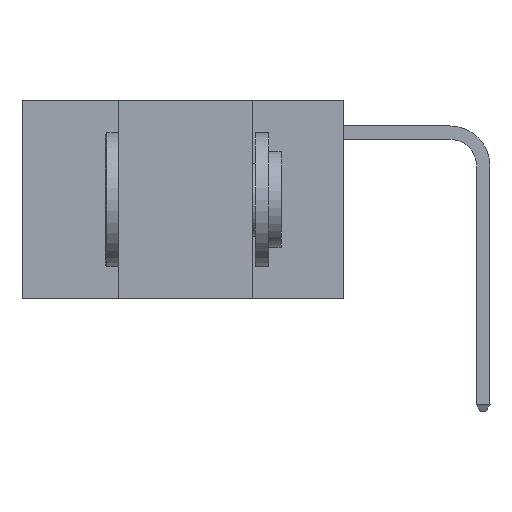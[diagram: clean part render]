
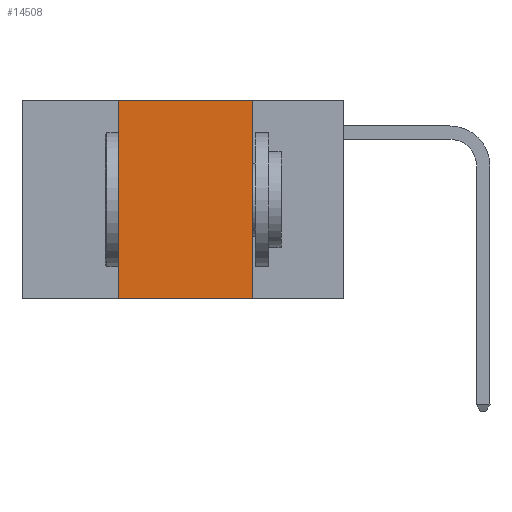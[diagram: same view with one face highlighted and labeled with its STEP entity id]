
A CAD part, left-side view. The second image highlights one B-rep face of the part: STEP entity #14508.
In plain terms, the highlighted planar face has unit normal (-1, 0, 0).
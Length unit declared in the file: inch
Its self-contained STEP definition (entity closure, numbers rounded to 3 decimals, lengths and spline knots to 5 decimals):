
#863 = DIRECTION ( 'NONE',  ( 0., -1., 0. ) ) ;
#2679 = LINE ( 'NONE', #19055, #10497 ) ;
#3425 = DIRECTION ( 'NONE',  ( 0., -1., 0. ) ) ;
#3497 = VECTOR ( 'NONE', #9899, 39.37008 ) ;
#4027 = CARTESIAN_POINT ( 'NONE',  ( 0., 0.6, -0.37 ) ) ;
#4130 = EDGE_LOOP ( 'NONE', ( #8446, #8509, #8854, #9112 ) ) ;
#4218 = VECTOR ( 'NONE', #3425, 39.37008 ) ;
#4928 = CARTESIAN_POINT ( 'NONE',  ( 0., 0.6, 0. ) ) ;
#6399 = DIRECTION ( 'NONE',  ( 0., 0., -1. ) ) ;
#6536 = CARTESIAN_POINT ( 'NONE',  ( 0., 0.17, 0. ) ) ;
#6576 = DIRECTION ( 'NONE',  ( 0., 0., -1. ) ) ;
#6963 = LINE ( 'NONE', #6536, #11026 ) ;
#8057 = PLANE ( 'NONE',  #15770 ) ;
#8110 = EDGE_CURVE ( 'NONE', #13884, #10195, #6963, .T. ) ;
#8275 = EDGE_CURVE ( 'NONE', #11967, #10195, #8441, .T. ) ;
#8441 = LINE ( 'NONE', #4027, #4218 ) ;
#8446 = ORIENTED_EDGE ( 'NONE', *, *, #8110, .F. ) ;
#8509 = ORIENTED_EDGE ( 'NONE', *, *, #11357, .F. ) ;
#8854 = ORIENTED_EDGE ( 'NONE', *, *, #15849, .F. ) ;
#9112 = ORIENTED_EDGE ( 'NONE', *, *, #8275, .T. ) ;
#9899 = DIRECTION ( 'NONE',  ( 0., 0., 1. ) ) ;
#10195 = VERTEX_POINT ( 'NONE', #19344 ) ;
#10497 = VECTOR ( 'NONE', #863, 39.37008 ) ;
#11026 = VECTOR ( 'NONE', #6399, 39.37008 ) ;
#11357 = EDGE_CURVE ( 'NONE', #13607, #13884, #2679, .T. ) ;
#11835 = LINE ( 'NONE', #12990, #3497 ) ;
#11910 = CARTESIAN_POINT ( 'NONE',  ( 0., 0.42, -0.37 ) ) ;
#11967 = VERTEX_POINT ( 'NONE', #11910 ) ;
#12990 = CARTESIAN_POINT ( 'NONE',  ( 0., 0.42, 0. ) ) ;
#13270 = FACE_OUTER_BOUND ( 'NONE', #4130, .T. ) ;
#13607 = VERTEX_POINT ( 'NONE', #18838 ) ;
#13884 = VERTEX_POINT ( 'NONE', #16610 ) ;
#14508 = ADVANCED_FACE ( 'NONE', ( #13270 ), #8057, .F. ) ;
#15619 = DIRECTION ( 'NONE',  ( 1., 0., 0. ) ) ;
#15770 = AXIS2_PLACEMENT_3D ( 'NONE', #4928, #15619, #6576 ) ;
#15849 = EDGE_CURVE ( 'NONE', #11967, #13607, #11835, .T. ) ;
#16610 = CARTESIAN_POINT ( 'NONE',  ( 0., 0.17, 0. ) ) ;
#18838 = CARTESIAN_POINT ( 'NONE',  ( 0., 0.42, 0. ) ) ;
#19055 = CARTESIAN_POINT ( 'NONE',  ( 0., 0.6, 0. ) ) ;
#19344 = CARTESIAN_POINT ( 'NONE',  ( 0., 0.17, -0.37 ) ) ;
